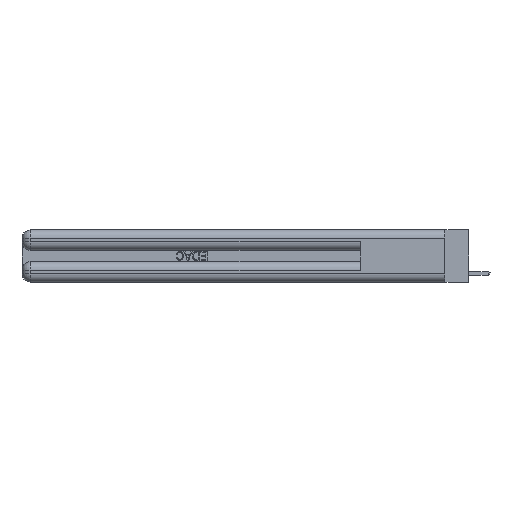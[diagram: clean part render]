
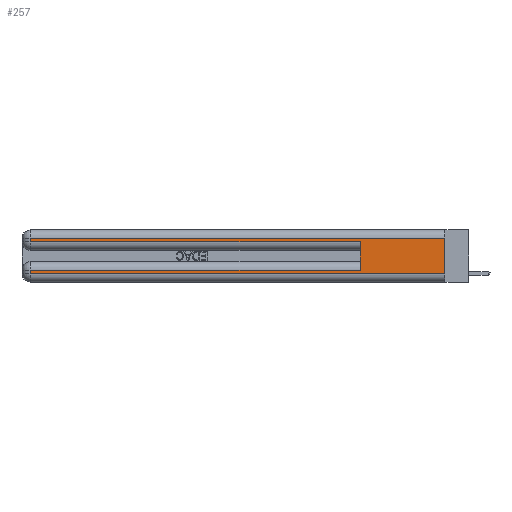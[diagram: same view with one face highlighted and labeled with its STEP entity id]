
A CAD part, left-side view. The second image highlights one B-rep face of the part: STEP entity #257.
In plain terms, the highlighted planar face has unit normal (-1, 0, 0).
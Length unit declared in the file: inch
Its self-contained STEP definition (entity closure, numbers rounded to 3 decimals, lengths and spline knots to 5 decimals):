
#257 = ADVANCED_FACE ( 'NONE', ( #20187 ), #15487, .F. ) ;
#347 = ORIENTED_EDGE ( 'NONE', *, *, #8110, .T. ) ;
#1413 = ORIENTED_EDGE ( 'NONE', *, *, #19569, .T. ) ;
#2026 = EDGE_CURVE ( 'NONE', #32622, #3725, #26513, .T. ) ;
#3085 = LINE ( 'NONE', #19233, #5482 ) ;
#3725 = VERTEX_POINT ( 'NONE', #5982 ) ;
#4235 = VECTOR ( 'NONE', #29792, 39.37008 ) ;
#5174 = ORIENTED_EDGE ( 'NONE', *, *, #27928, .T. ) ;
#5482 = VECTOR ( 'NONE', #19560, 39.37008 ) ;
#5720 = VERTEX_POINT ( 'NONE', #22370 ) ;
#5982 = CARTESIAN_POINT ( 'NONE',  ( 0., 2.94, 0.285 ) ) ;
#6240 = CARTESIAN_POINT ( 'NONE',  ( 0., 2.94, 0.06 ) ) ;
#7044 = VERTEX_POINT ( 'NONE', #26845 ) ;
#7075 = DIRECTION ( 'NONE',  ( 0., 0., -1. ) ) ;
#7963 = VECTOR ( 'NONE', #7075, 39.37008 ) ;
#8110 = EDGE_CURVE ( 'NONE', #3725, #13889, #32834, .T. ) ;
#8956 = CARTESIAN_POINT ( 'NONE',  ( 0., 0., 0.085 ) ) ;
#10407 = CARTESIAN_POINT ( 'NONE',  ( 0., 0., 0.37 ) ) ;
#11503 = LINE ( 'NONE', #23592, #21149 ) ;
#12264 = CARTESIAN_POINT ( 'NONE',  ( 0., 2.94, 0.31 ) ) ;
#12913 = DIRECTION ( 'NONE',  ( 0., 0., -1. ) ) ;
#12952 = VECTOR ( 'NONE', #30770, 39.37008 ) ;
#13513 = CARTESIAN_POINT ( 'NONE',  ( 0., 0.6, 0.145 ) ) ;
#13889 = VERTEX_POINT ( 'NONE', #21434 ) ;
#14067 = CARTESIAN_POINT ( 'NONE',  ( 0., 0., 0.285 ) ) ;
#14423 = EDGE_LOOP ( 'NONE', ( #24612, #1413, #23469, #347, #15426, #32279, #5174, #18282 ) ) ;
#15426 = ORIENTED_EDGE ( 'NONE', *, *, #29871, .F. ) ;
#15487 = PLANE ( 'NONE',  #29104 ) ;
#15596 = DIRECTION ( 'NONE',  ( 1., 0., 0. ) ) ;
#16231 = VERTEX_POINT ( 'NONE', #30884 ) ;
#16303 = EDGE_CURVE ( 'NONE', #7044, #16231, #17342, .T. ) ;
#16506 = LINE ( 'NONE', #8956, #26984 ) ;
#16738 = DIRECTION ( 'NONE',  ( 0., 1., 0. ) ) ;
#17157 = CARTESIAN_POINT ( 'NONE',  ( 0., 0., 0.31 ) ) ;
#17342 = LINE ( 'NONE', #10407, #12952 ) ;
#18108 = VECTOR ( 'NONE', #32686, 39.37008 ) ;
#18282 = ORIENTED_EDGE ( 'NONE', *, *, #31831, .T. ) ;
#19233 = CARTESIAN_POINT ( 'NONE',  ( 0., 2.94, 0.37 ) ) ;
#19265 = VERTEX_POINT ( 'NONE', #6240 ) ;
#19463 = EDGE_CURVE ( 'NONE', #21238, #5720, #16506, .T. ) ;
#19560 = DIRECTION ( 'NONE',  ( 0., 0., -1. ) ) ;
#19569 = EDGE_CURVE ( 'NONE', #7044, #32622, #20546, .T. ) ;
#20187 = FACE_OUTER_BOUND ( 'NONE', #14423, .T. ) ;
#20546 = LINE ( 'NONE', #17157, #18108 ) ;
#20672 = CARTESIAN_POINT ( 'NONE',  ( 0., 0., 0.37 ) ) ;
#21149 = VECTOR ( 'NONE', #26208, 39.37008 ) ;
#21238 = VERTEX_POINT ( 'NONE', #28035 ) ;
#21434 = CARTESIAN_POINT ( 'NONE',  ( 0., 0.6, 0.285 ) ) ;
#22370 = CARTESIAN_POINT ( 'NONE',  ( 0., 2.94, 0.085 ) ) ;
#23469 = ORIENTED_EDGE ( 'NONE', *, *, #2026, .T. ) ;
#23592 = CARTESIAN_POINT ( 'NONE',  ( 0., 0., 0.06 ) ) ;
#23829 = DIRECTION ( 'NONE',  ( 0., 0., 1. ) ) ;
#24612 = ORIENTED_EDGE ( 'NONE', *, *, #16303, .F. ) ;
#26208 = DIRECTION ( 'NONE',  ( 0., -1., 0. ) ) ;
#26488 = VECTOR ( 'NONE', #23829, 39.37008 ) ;
#26513 = LINE ( 'NONE', #33206, #7963 ) ;
#26845 = CARTESIAN_POINT ( 'NONE',  ( 0., 0., 0.31 ) ) ;
#26984 = VECTOR ( 'NONE', #16738, 39.37008 ) ;
#27928 = EDGE_CURVE ( 'NONE', #5720, #19265, #3085, .T. ) ;
#28035 = CARTESIAN_POINT ( 'NONE',  ( 0., 0.6, 0.085 ) ) ;
#28819 = LINE ( 'NONE', #13513, #26488 ) ;
#29104 = AXIS2_PLACEMENT_3D ( 'NONE', #20672, #15596, #12913 ) ;
#29792 = DIRECTION ( 'NONE',  ( 0., -1., 0. ) ) ;
#29871 = EDGE_CURVE ( 'NONE', #21238, #13889, #28819, .T. ) ;
#30770 = DIRECTION ( 'NONE',  ( 0., 0., -1. ) ) ;
#30884 = CARTESIAN_POINT ( 'NONE',  ( 0., 0., 0.06 ) ) ;
#31831 = EDGE_CURVE ( 'NONE', #19265, #16231, #11503, .T. ) ;
#32279 = ORIENTED_EDGE ( 'NONE', *, *, #19463, .T. ) ;
#32622 = VERTEX_POINT ( 'NONE', #12264 ) ;
#32686 = DIRECTION ( 'NONE',  ( 0., 1., 0. ) ) ;
#32834 = LINE ( 'NONE', #14067, #4235 ) ;
#33206 = CARTESIAN_POINT ( 'NONE',  ( 0., 2.94, 0.37 ) ) ;
